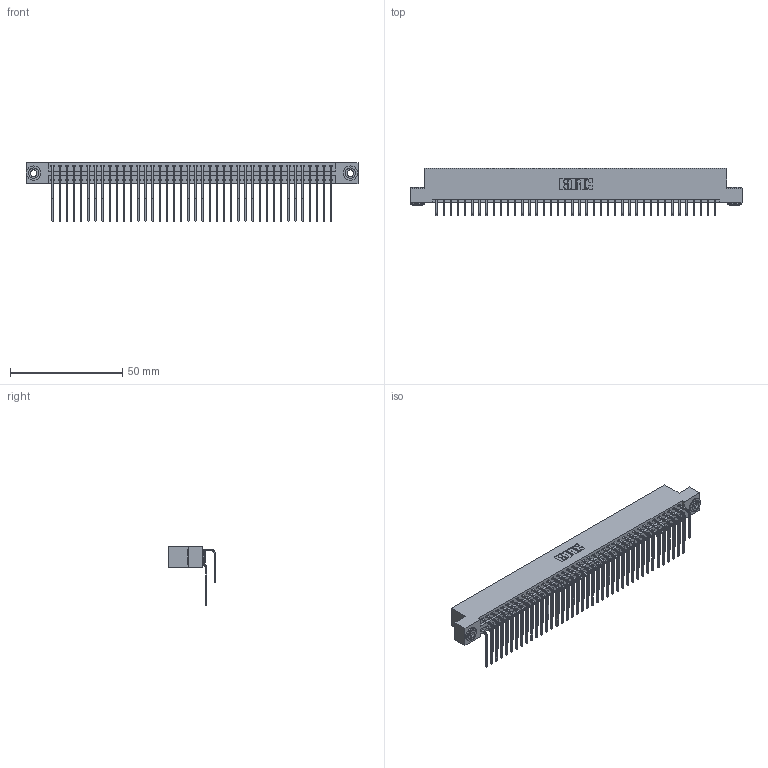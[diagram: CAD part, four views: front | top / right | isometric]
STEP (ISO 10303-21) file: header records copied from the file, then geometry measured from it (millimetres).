
FILE_DESCRIPTION (( 'STEP AP203' ), '1' );
FILE_NAME ('396-080-559-203.STEP', '2018-09-09T21:43:46', ( '' ), ( '' ), 'SwSTEP 2.0', 'SolidWorks 2016', '' );
FILE_SCHEMA (( 'CONFIG_CONTROL_DESIGN' ));
Length unit declared in the file: inch
Products named in the file (5): 346 Part_Flush Mounting Lugs - 0.156 Dia-TH; 345-292-001_558 559 Tail - 1; 345-292-001_559 Tail - 2; 345-250-002_345-250-002-102; 396-080-559-203
Assembly tree (83 placements, depth 2):
  396-080-559-203
    346 Part_Flush Mounting Lugs - 0.156 Dia-TH
    345-292-001_558 559 Tail - 1  x40
    345-292-001_559 Tail - 2  x40
    345-250-002_345-250-002-102  x2
Bounding box: 147.57 x 20.89 x 26.16 mm (x, y, z)
Volume: 14855.7 mm3; surface area: 22816.8 mm2
Topology: 83 solids, 83 shells, 4480 faces, 13285 edges, 8746 vertices
Faces by surface type: plane 3046, cylinder 1426, cone 8
Entity records: 28808 total; most frequent: CARTESIAN_POINT 4778, ORIENTED_EDGE 4654, DIRECTION 4265, EDGE_CURVE 2327, VECTOR 1971, LINE 1971, VERTEX_POINT 1546, AXIS2_PLACEMENT_3D 1147
